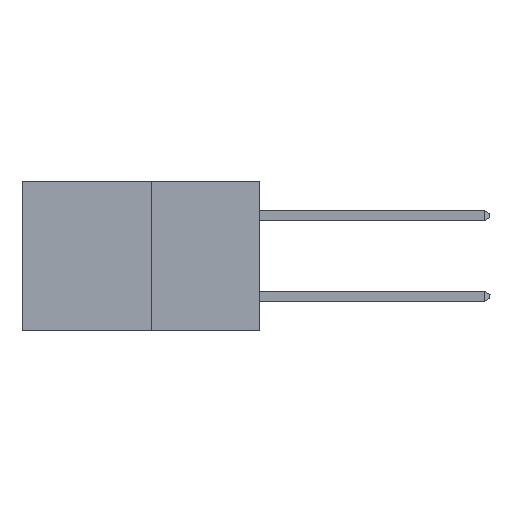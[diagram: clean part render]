
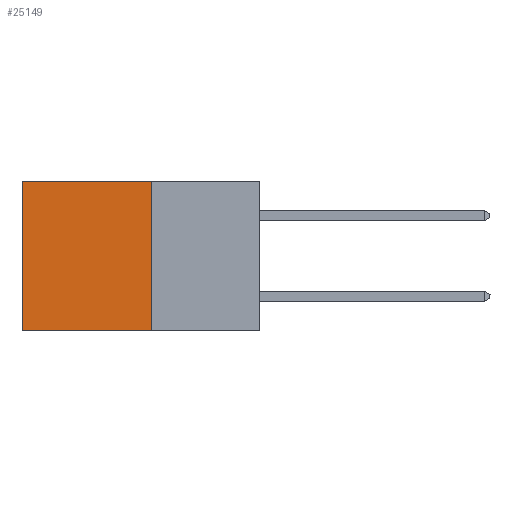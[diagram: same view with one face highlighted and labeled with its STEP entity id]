
A CAD part, left-side view. The second image highlights one B-rep face of the part: STEP entity #25149.
In plain terms, the highlighted planar face has unit normal (-1, 0, 0).
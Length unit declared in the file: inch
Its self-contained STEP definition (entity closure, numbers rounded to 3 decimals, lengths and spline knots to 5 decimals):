
#198 = VECTOR ( 'NONE', #15757, 39.37008 ) ;
#1151 = DIRECTION ( 'NONE',  ( 0., 1., 0. ) ) ;
#1819 = ORIENTED_EDGE ( 'NONE', *, *, #4861, .F. ) ;
#2358 = CARTESIAN_POINT ( 'NONE',  ( 0.277, 0.27, 0. ) ) ;
#3125 = ORIENTED_EDGE ( 'NONE', *, *, #7277, .F. ) ;
#3745 = VERTEX_POINT ( 'NONE', #2358 ) ;
#4489 = ORIENTED_EDGE ( 'NONE', *, *, #6458, .T. ) ;
#4780 = CARTESIAN_POINT ( 'NONE',  ( 0.277, 0.27, -0.37 ) ) ;
#4861 = EDGE_CURVE ( 'NONE', #3745, #20069, #9370, .T. ) ;
#5169 = CARTESIAN_POINT ( 'NONE',  ( 0.277, 0.59, 0. ) ) ;
#5444 = VECTOR ( 'NONE', #25199, 39.37008 ) ;
#5778 = EDGE_CURVE ( 'NONE', #17618, #6659, #15448, .T. ) ;
#6338 = LINE ( 'NONE', #8894, #198 ) ;
#6458 = EDGE_CURVE ( 'NONE', #3745, #17618, #6338, .T. ) ;
#6659 = VERTEX_POINT ( 'NONE', #21689 ) ;
#6851 = CARTESIAN_POINT ( 'NONE',  ( 0.277, 0.27, -0.37 ) ) ;
#7277 = EDGE_CURVE ( 'NONE', #20069, #6659, #14865, .T. ) ;
#8875 = DIRECTION ( 'NONE',  ( 0., 0., -1. ) ) ;
#8894 = CARTESIAN_POINT ( 'NONE',  ( 0.277, 0.27, 0. ) ) ;
#9370 = LINE ( 'NONE', #23079, #5444 ) ;
#9796 = FACE_OUTER_BOUND ( 'NONE', #24706, .T. ) ;
#14429 = CARTESIAN_POINT ( 'NONE',  ( 0.277, 0.59, -0.37 ) ) ;
#14865 = LINE ( 'NONE', #4780, #19460 ) ;
#15448 = LINE ( 'NONE', #14429, #20693 ) ;
#15757 = DIRECTION ( 'NONE',  ( 0., 1., 0. ) ) ;
#17618 = VERTEX_POINT ( 'NONE', #5169 ) ;
#18324 = DIRECTION ( 'NONE',  ( 0., 0., -1. ) ) ;
#19460 = VECTOR ( 'NONE', #1151, 39.37008 ) ;
#19760 = ORIENTED_EDGE ( 'NONE', *, *, #5778, .T. ) ;
#20069 = VERTEX_POINT ( 'NONE', #24369 ) ;
#20693 = VECTOR ( 'NONE', #18324, 39.37008 ) ;
#20748 = DIRECTION ( 'NONE',  ( 1., 0., 0. ) ) ;
#21689 = CARTESIAN_POINT ( 'NONE',  ( 0.277, 0.59, -0.37 ) ) ;
#22627 = PLANE ( 'NONE',  #24457 ) ;
#23079 = CARTESIAN_POINT ( 'NONE',  ( 0.277, 0.27, -0.37 ) ) ;
#24369 = CARTESIAN_POINT ( 'NONE',  ( 0.277, 0.27, -0.37 ) ) ;
#24457 = AXIS2_PLACEMENT_3D ( 'NONE', #6851, #20748, #8875 ) ;
#24706 = EDGE_LOOP ( 'NONE', ( #19760, #3125, #1819, #4489 ) ) ;
#25149 = ADVANCED_FACE ( 'NONE', ( #9796 ), #22627, .F. ) ;
#25199 = DIRECTION ( 'NONE',  ( 0., 0., -1. ) ) ;
